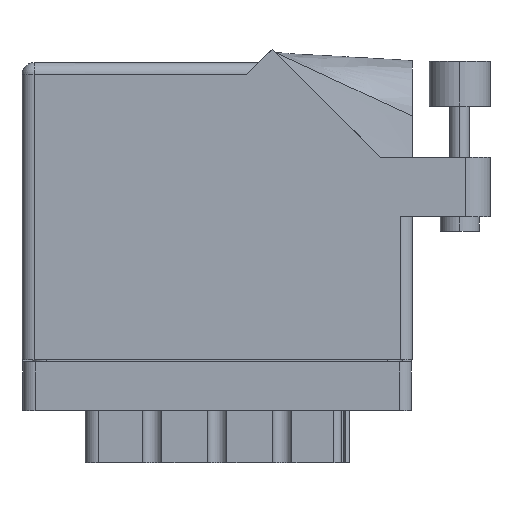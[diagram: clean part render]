
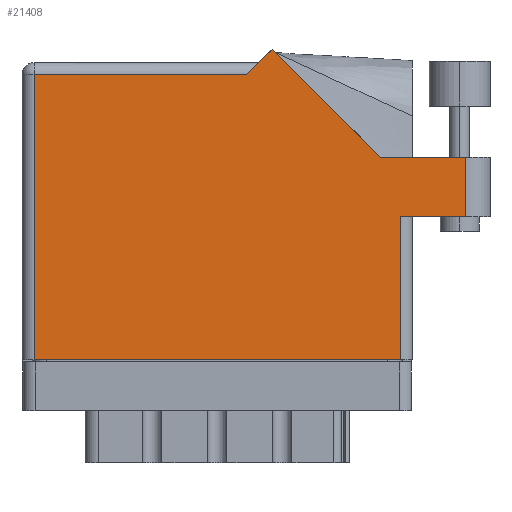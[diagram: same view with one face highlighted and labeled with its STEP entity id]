
A CAD part, front view. The second image highlights one B-rep face of the part: STEP entity #21408.
In plain terms, the highlighted face is planar.
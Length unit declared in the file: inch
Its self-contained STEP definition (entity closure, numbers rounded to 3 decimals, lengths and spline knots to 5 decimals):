
#767 = CARTESIAN_POINT ( 'NONE',  ( 2.285, 1.044, 0. ) ) ;
#1641 = LINE ( 'NONE', #19757, #16865 ) ;
#1871 = CARTESIAN_POINT ( 'NONE',  ( 1.28771, 1.60071, 0. ) ) ;
#3083 = CARTESIAN_POINT ( 'NONE',  ( 1.948, 0.737, 0. ) ) ;
#3971 = DIRECTION ( 'NONE',  ( -0.707, -0.707, 0. ) ) ;
#4009 = ORIENTED_EDGE ( 'NONE', *, *, #16940, .T. ) ;
#4090 = AXIS2_PLACEMENT_3D ( 'NONE', #23571, #10757, #23344 ) ;
#4583 = VECTOR ( 'NONE', #32878, 39.37008 ) ;
#5314 = ORIENTED_EDGE ( 'NONE', *, *, #21663, .T. ) ;
#5356 = PLANE ( 'NONE',  #4090 ) ;
#5448 = VECTOR ( 'NONE', #33233, 39.37008 ) ;
#6026 = CARTESIAN_POINT ( 'NONE',  ( 1.155, 1.468, 0. ) ) ;
#6473 = LINE ( 'NONE', #29542, #22945 ) ;
#6715 = CARTESIAN_POINT ( 'NONE',  ( 0., 0., 0. ) ) ;
#6879 = VECTOR ( 'NONE', #32249, 39.37008 ) ;
#7052 = CARTESIAN_POINT ( 'NONE',  ( 0.062, 0., 0. ) ) ;
#7060 = LINE ( 'NONE', #15202, #5448 ) ;
#7097 = ORIENTED_EDGE ( 'NONE', *, *, #24931, .T. ) ;
#7674 = VECTOR ( 'NONE', #26034, 39.37008 ) ;
#8822 = CARTESIAN_POINT ( 'NONE',  ( 1.84442, 1.044, 0. ) ) ;
#9211 = VERTEX_POINT ( 'NONE', #6026 ) ;
#10757 = DIRECTION ( 'NONE',  ( 0., 0., -1. ) ) ;
#11012 = EDGE_CURVE ( 'NONE', #19242, #19819, #31783, .T. ) ;
#11565 = VERTEX_POINT ( 'NONE', #767 ) ;
#11986 = LINE ( 'NONE', #7052, #33306 ) ;
#13708 = EDGE_CURVE ( 'NONE', #19819, #15432, #7060, .T. ) ;
#14016 = DIRECTION ( 'NONE',  ( -1., 0., 0. ) ) ;
#14334 = ORIENTED_EDGE ( 'NONE', *, *, #28701, .T. ) ;
#14787 = DIRECTION ( 'NONE',  ( 0., -1., 0. ) ) ;
#15202 = CARTESIAN_POINT ( 'NONE',  ( 2.01, 0.737, 0. ) ) ;
#15432 = VERTEX_POINT ( 'NONE', #19447 ) ;
#16257 = EDGE_CURVE ( 'NONE', #15432, #11565, #28153, .T. ) ;
#16865 = VECTOR ( 'NONE', #27883, 39.37008 ) ;
#16940 = EDGE_CURVE ( 'NONE', #20734, #30279, #11986, .T. ) ;
#17380 = VECTOR ( 'NONE', #14016, 39.37008 ) ;
#19242 = VERTEX_POINT ( 'NONE', #25679 ) ;
#19332 = EDGE_LOOP ( 'NONE', ( #31832, #28656, #28358, #14334, #5314, #7097, #4009, #23006, #29717 ) ) ;
#19447 = CARTESIAN_POINT ( 'NONE',  ( 2.285, 0.737, 0. ) ) ;
#19757 = CARTESIAN_POINT ( 'NONE',  ( 1.84442, 1.044, 0. ) ) ;
#19819 = VERTEX_POINT ( 'NONE', #28485 ) ;
#20670 = EDGE_CURVE ( 'NONE', #30279, #19242, #27419, .T. ) ;
#20734 = VERTEX_POINT ( 'NONE', #26751 ) ;
#21408 = ADVANCED_FACE ( 'NONE', ( #25403 ), #5356, .F. ) ;
#21663 = EDGE_CURVE ( 'NONE', #29186, #9211, #6473, .T. ) ;
#22945 = VECTOR ( 'NONE', #3971, 39.37008 ) ;
#23006 = ORIENTED_EDGE ( 'NONE', *, *, #20670, .T. ) ;
#23344 = DIRECTION ( 'NONE',  ( -1., 0., 0. ) ) ;
#23571 = CARTESIAN_POINT ( 'NONE',  ( 0., 1.53, 0. ) ) ;
#24833 = CARTESIAN_POINT ( 'NONE',  ( 0.062, 0., 0. ) ) ;
#24875 = VERTEX_POINT ( 'NONE', #8822 ) ;
#24897 = CARTESIAN_POINT ( 'NONE',  ( 0., 1.468, 0. ) ) ;
#24931 = EDGE_CURVE ( 'NONE', #9211, #20734, #25125, .T. ) ;
#25125 = LINE ( 'NONE', #24897, #4583 ) ;
#25403 = FACE_OUTER_BOUND ( 'NONE', #19332, .T. ) ;
#25679 = CARTESIAN_POINT ( 'NONE',  ( 1.948, 0., 0. ) ) ;
#26034 = DIRECTION ( 'NONE',  ( 0., 1., 0. ) ) ;
#26751 = CARTESIAN_POINT ( 'NONE',  ( 0.062, 1.468, 0. ) ) ;
#26861 = CARTESIAN_POINT ( 'NONE',  ( 2.41, 1.044, 0. ) ) ;
#27099 = LINE ( 'NONE', #26861, #17380 ) ;
#27302 = EDGE_CURVE ( 'NONE', #11565, #24875, #27099, .T. ) ;
#27419 = LINE ( 'NONE', #6715, #6879 ) ;
#27797 = DIRECTION ( 'NONE',  ( 0., 1., 0. ) ) ;
#27883 = DIRECTION ( 'NONE',  ( -0.707, 0.707, 0. ) ) ;
#28153 = LINE ( 'NONE', #32758, #29362 ) ;
#28358 = ORIENTED_EDGE ( 'NONE', *, *, #27302, .T. ) ;
#28485 = CARTESIAN_POINT ( 'NONE',  ( 1.948, 0.737, 0. ) ) ;
#28656 = ORIENTED_EDGE ( 'NONE', *, *, #16257, .T. ) ;
#28701 = EDGE_CURVE ( 'NONE', #24875, #29186, #1641, .T. ) ;
#29186 = VERTEX_POINT ( 'NONE', #1871 ) ;
#29362 = VECTOR ( 'NONE', #27797, 39.37008 ) ;
#29542 = CARTESIAN_POINT ( 'NONE',  ( 1.217, 1.53, 0. ) ) ;
#29717 = ORIENTED_EDGE ( 'NONE', *, *, #11012, .T. ) ;
#30279 = VERTEX_POINT ( 'NONE', #24833 ) ;
#31783 = LINE ( 'NONE', #3083, #7674 ) ;
#31832 = ORIENTED_EDGE ( 'NONE', *, *, #13708, .T. ) ;
#32249 = DIRECTION ( 'NONE',  ( 1., 0., 0. ) ) ;
#32758 = CARTESIAN_POINT ( 'NONE',  ( 2.285, 1.044, 0. ) ) ;
#32878 = DIRECTION ( 'NONE',  ( -1., 0., 0. ) ) ;
#33233 = DIRECTION ( 'NONE',  ( 1., 0., 0. ) ) ;
#33306 = VECTOR ( 'NONE', #14787, 39.37008 ) ;
